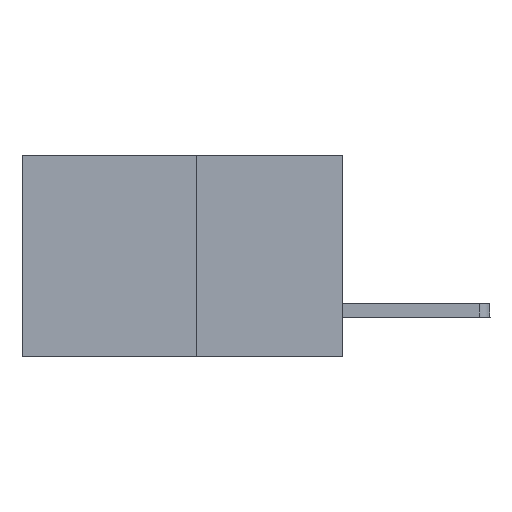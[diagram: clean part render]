
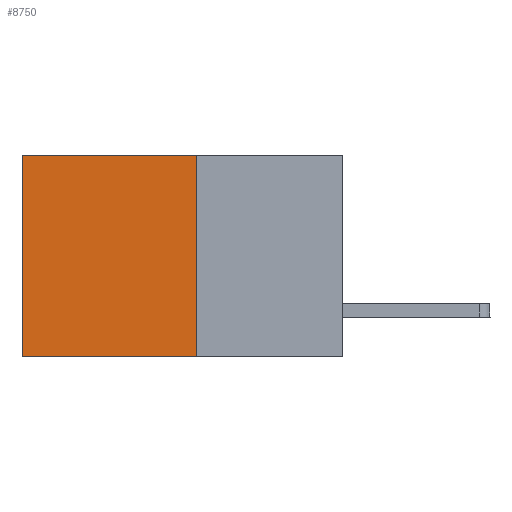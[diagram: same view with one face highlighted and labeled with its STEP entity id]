
A CAD part, left-side view. The second image highlights one B-rep face of the part: STEP entity #8750.
In plain terms, the highlighted planar face has unit normal (-1, 0, 0).
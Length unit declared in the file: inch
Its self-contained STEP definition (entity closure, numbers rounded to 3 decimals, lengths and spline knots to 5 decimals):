
#121 = CARTESIAN_POINT ( 'NONE',  ( 0.277, 0.27, -0.37 ) ) ;
#195 = EDGE_CURVE ( 'NONE', #7844, #5188, #3713, .T. ) ;
#262 = CARTESIAN_POINT ( 'NONE',  ( 0.277, 0.27, -0.37 ) ) ;
#966 = DIRECTION ( 'NONE',  ( 0., 0., -1. ) ) ;
#2104 = EDGE_CURVE ( 'NONE', #2488, #4491, #2364, .T. ) ;
#2154 = CARTESIAN_POINT ( 'NONE',  ( 0.277, 0.27, -0.37 ) ) ;
#2364 = LINE ( 'NONE', #121, #2806 ) ;
#2407 = PLANE ( 'NONE',  #3628 ) ;
#2488 = VERTEX_POINT ( 'NONE', #3258 ) ;
#2586 = ORIENTED_EDGE ( 'NONE', *, *, #195, .T. ) ;
#2806 = VECTOR ( 'NONE', #3948, 39.37008 ) ;
#2840 = EDGE_CURVE ( 'NONE', #2488, #7844, #3894, .T. ) ;
#2935 = VECTOR ( 'NONE', #7854, 39.37008 ) ;
#3258 = CARTESIAN_POINT ( 'NONE',  ( 0.277, 0.27, 0. ) ) ;
#3628 = AXIS2_PLACEMENT_3D ( 'NONE', #262, #8547, #966 ) ;
#3713 = LINE ( 'NONE', #7431, #5214 ) ;
#3894 = LINE ( 'NONE', #4787, #6246 ) ;
#3948 = DIRECTION ( 'NONE',  ( 0., 0., -1. ) ) ;
#4193 = ORIENTED_EDGE ( 'NONE', *, *, #6797, .F. ) ;
#4260 = ORIENTED_EDGE ( 'NONE', *, *, #2104, .F. ) ;
#4491 = VERTEX_POINT ( 'NONE', #2154 ) ;
#4787 = CARTESIAN_POINT ( 'NONE',  ( 0.277, 0.27, 0. ) ) ;
#5188 = VERTEX_POINT ( 'NONE', #7686 ) ;
#5214 = VECTOR ( 'NONE', #6786, 39.37008 ) ;
#5576 = LINE ( 'NONE', #9336, #2935 ) ;
#6169 = FACE_OUTER_BOUND ( 'NONE', #9670, .T. ) ;
#6219 = CARTESIAN_POINT ( 'NONE',  ( 0.277, 0.59, 0. ) ) ;
#6246 = VECTOR ( 'NONE', #6914, 39.37008 ) ;
#6786 = DIRECTION ( 'NONE',  ( 0., 0., -1. ) ) ;
#6797 = EDGE_CURVE ( 'NONE', #4491, #5188, #5576, .T. ) ;
#6914 = DIRECTION ( 'NONE',  ( 0., 1., 0. ) ) ;
#7431 = CARTESIAN_POINT ( 'NONE',  ( 0.277, 0.59, -0.37 ) ) ;
#7686 = CARTESIAN_POINT ( 'NONE',  ( 0.277, 0.59, -0.37 ) ) ;
#7844 = VERTEX_POINT ( 'NONE', #6219 ) ;
#7854 = DIRECTION ( 'NONE',  ( 0., 1., 0. ) ) ;
#8109 = ORIENTED_EDGE ( 'NONE', *, *, #2840, .T. ) ;
#8547 = DIRECTION ( 'NONE',  ( 1., 0., 0. ) ) ;
#8750 = ADVANCED_FACE ( 'NONE', ( #6169 ), #2407, .F. ) ;
#9336 = CARTESIAN_POINT ( 'NONE',  ( 0.277, 0.27, -0.37 ) ) ;
#9670 = EDGE_LOOP ( 'NONE', ( #2586, #4193, #4260, #8109 ) ) ;
